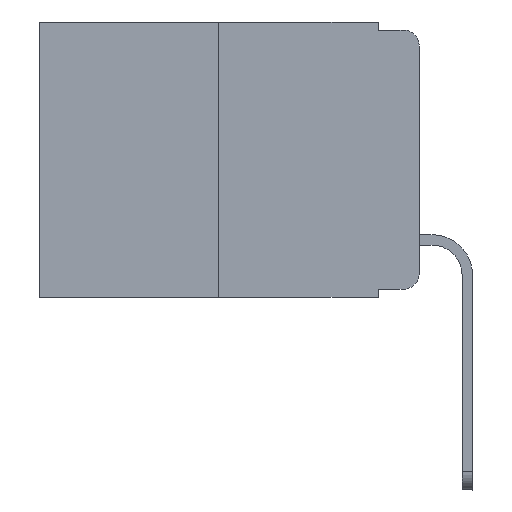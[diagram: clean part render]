
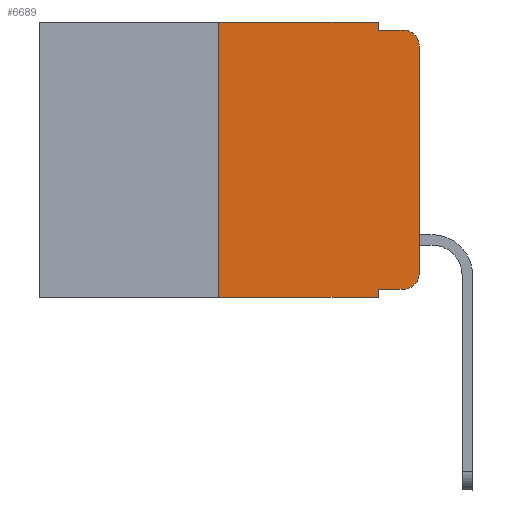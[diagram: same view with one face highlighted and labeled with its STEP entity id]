
A CAD part, left-side view. The second image highlights one B-rep face of the part: STEP entity #6689.
In plain terms, the highlighted planar face has unit normal (-1, 0, 0).
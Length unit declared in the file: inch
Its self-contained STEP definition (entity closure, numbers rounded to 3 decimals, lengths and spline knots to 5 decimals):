
#243 = ORIENTED_EDGE ( 'NONE', *, *, #19331, .F. ) ;
#561 = CARTESIAN_POINT ( 'NONE',  ( 0., 0.051, 0. ) ) ;
#602 = CARTESIAN_POINT ( 'NONE',  ( 0., 0.02, -0.333 ) ) ;
#1214 = CARTESIAN_POINT ( 'NONE',  ( 0., 0.051, -0.333 ) ) ;
#1800 = CARTESIAN_POINT ( 'NONE',  ( 0., 0.25, -0.343 ) ) ;
#2086 = VECTOR ( 'NONE', #14209, 39.37008 ) ;
#2180 = LINE ( 'NONE', #3840, #2086 ) ;
#2734 = LINE ( 'NONE', #9473, #9349 ) ;
#2852 = DIRECTION ( 'NONE',  ( 0., -1., 0. ) ) ;
#3144 = VERTEX_POINT ( 'NONE', #11493 ) ;
#3840 = CARTESIAN_POINT ( 'NONE',  ( 0., 0.051, -0.01 ) ) ;
#4466 = CARTESIAN_POINT ( 'NONE',  ( 0., 0.051, -0.333 ) ) ;
#4474 = LINE ( 'NONE', #9321, #17588 ) ;
#4790 = ORIENTED_EDGE ( 'NONE', *, *, #19199, .F. ) ;
#5009 = VERTEX_POINT ( 'NONE', #18553 ) ;
#5199 = LINE ( 'NONE', #20678, #15040 ) ;
#5348 = AXIS2_PLACEMENT_3D ( 'NONE', #19692, #21131, #15921 ) ;
#6081 = VERTEX_POINT ( 'NONE', #602 ) ;
#6203 = PLANE ( 'NONE',  #5348 ) ;
#6318 = VERTEX_POINT ( 'NONE', #10077 ) ;
#6421 = VERTEX_POINT ( 'NONE', #21821 ) ;
#6426 = VERTEX_POINT ( 'NONE', #1800 ) ;
#6503 = ORIENTED_EDGE ( 'NONE', *, *, #16864, .T. ) ;
#6535 = CARTESIAN_POINT ( 'NONE',  ( 0., 0.25, 0. ) ) ;
#6583 = VECTOR ( 'NONE', #19431, 39.37008 ) ;
#6598 = EDGE_CURVE ( 'NONE', #7490, #6318, #20172, .T. ) ;
#6689 = ADVANCED_FACE ( 'NONE', ( #9181 ), #6203, .F. ) ;
#7224 = ORIENTED_EDGE ( 'NONE', *, *, #17387, .T. ) ;
#7490 = VERTEX_POINT ( 'NONE', #12988 ) ;
#7732 = DIRECTION ( 'NONE',  ( 0., 0., -1. ) ) ;
#8122 = ORIENTED_EDGE ( 'NONE', *, *, #9106, .T. ) ;
#8833 = ORIENTED_EDGE ( 'NONE', *, *, #16316, .F. ) ;
#9032 = LINE ( 'NONE', #10810, #6583 ) ;
#9106 = EDGE_CURVE ( 'NONE', #6426, #5009, #2734, .T. ) ;
#9181 = FACE_OUTER_BOUND ( 'NONE', #17585, .T. ) ;
#9239 = DIRECTION ( 'NONE',  ( -1., 0., 0. ) ) ;
#9275 = CARTESIAN_POINT ( 'NONE',  ( 0., 0.051, 0. ) ) ;
#9321 = CARTESIAN_POINT ( 'NONE',  ( 0., 0., 0. ) ) ;
#9349 = VECTOR ( 'NONE', #16213, 39.37008 ) ;
#9374 = VECTOR ( 'NONE', #13187, 39.37008 ) ;
#9473 = CARTESIAN_POINT ( 'NONE',  ( 0., 0.473, -0.343 ) ) ;
#10077 = CARTESIAN_POINT ( 'NONE',  ( 0., 0.02, -0.01 ) ) ;
#10615 = ORIENTED_EDGE ( 'NONE', *, *, #12218, .T. ) ;
#10810 = CARTESIAN_POINT ( 'NONE',  ( 0., 0.051, 0. ) ) ;
#10839 = LINE ( 'NONE', #9275, #20372 ) ;
#11035 = ORIENTED_EDGE ( 'NONE', *, *, #6598, .T. ) ;
#11063 = CARTESIAN_POINT ( 'NONE',  ( 0., 0.02, -0.03 ) ) ;
#11137 = VERTEX_POINT ( 'NONE', #4466 ) ;
#11349 = DIRECTION ( 'NONE',  ( 0., 0., -1. ) ) ;
#11408 = LINE ( 'NONE', #6535, #9374 ) ;
#11493 = CARTESIAN_POINT ( 'NONE',  ( 0., 0., -0.313 ) ) ;
#12218 = EDGE_CURVE ( 'NONE', #11137, #6081, #16334, .T. ) ;
#12302 = ORIENTED_EDGE ( 'NONE', *, *, #20668, .F. ) ;
#12988 = CARTESIAN_POINT ( 'NONE',  ( 0., 0., -0.03 ) ) ;
#13187 = DIRECTION ( 'NONE',  ( 0., 0., 1. ) ) ;
#14037 = AXIS2_PLACEMENT_3D ( 'NONE', #17649, #9239, #11349 ) ;
#14209 = DIRECTION ( 'NONE',  ( 0., -1., 0. ) ) ;
#14362 = DIRECTION ( 'NONE',  ( 0., 0., -1. ) ) ;
#15040 = VECTOR ( 'NONE', #20454, 39.37008 ) ;
#15797 = CIRCLE ( 'NONE', #14037, 0.02 ) ;
#15921 = DIRECTION ( 'NONE',  ( 0., 0., -1. ) ) ;
#16213 = DIRECTION ( 'NONE',  ( 0., -1., 0. ) ) ;
#16297 = VECTOR ( 'NONE', #2852, 39.37008 ) ;
#16316 = EDGE_CURVE ( 'NONE', #6421, #6318, #2180, .T. ) ;
#16334 = LINE ( 'NONE', #1214, #16297 ) ;
#16864 = EDGE_CURVE ( 'NONE', #6081, #3144, #15797, .T. ) ;
#17387 = EDGE_CURVE ( 'NONE', #3144, #7490, #4474, .T. ) ;
#17585 = EDGE_LOOP ( 'NONE', ( #7224, #11035, #8833, #12302, #243, #4790, #8122, #18000, #10615, #6503 ) ) ;
#17588 = VECTOR ( 'NONE', #21167, 39.37008 ) ;
#17649 = CARTESIAN_POINT ( 'NONE',  ( 0., 0.02, -0.313 ) ) ;
#17808 = VERTEX_POINT ( 'NONE', #21362 ) ;
#18000 = ORIENTED_EDGE ( 'NONE', *, *, #19799, .F. ) ;
#18037 = VERTEX_POINT ( 'NONE', #561 ) ;
#18553 = CARTESIAN_POINT ( 'NONE',  ( 0., 0.051, -0.343 ) ) ;
#19199 = EDGE_CURVE ( 'NONE', #6426, #17808, #11408, .T. ) ;
#19331 = EDGE_CURVE ( 'NONE', #17808, #18037, #5199, .T. ) ;
#19431 = DIRECTION ( 'NONE',  ( 0., 0., -1. ) ) ;
#19584 = DIRECTION ( 'NONE',  ( -1., 0., 0. ) ) ;
#19692 = CARTESIAN_POINT ( 'NONE',  ( 0., 0.473, 0. ) ) ;
#19799 = EDGE_CURVE ( 'NONE', #11137, #5009, #9032, .T. ) ;
#20172 = CIRCLE ( 'NONE', #20517, 0.02 ) ;
#20372 = VECTOR ( 'NONE', #14362, 39.37008 ) ;
#20454 = DIRECTION ( 'NONE',  ( 0., -1., 0. ) ) ;
#20517 = AXIS2_PLACEMENT_3D ( 'NONE', #11063, #19584, #7732 ) ;
#20668 = EDGE_CURVE ( 'NONE', #18037, #6421, #10839, .T. ) ;
#20678 = CARTESIAN_POINT ( 'NONE',  ( 0., 0.473, 0. ) ) ;
#21131 = DIRECTION ( 'NONE',  ( 1., 0., 0. ) ) ;
#21167 = DIRECTION ( 'NONE',  ( 0., 0., 1. ) ) ;
#21362 = CARTESIAN_POINT ( 'NONE',  ( 0., 0.25, 0. ) ) ;
#21821 = CARTESIAN_POINT ( 'NONE',  ( 0., 0.051, -0.01 ) ) ;
